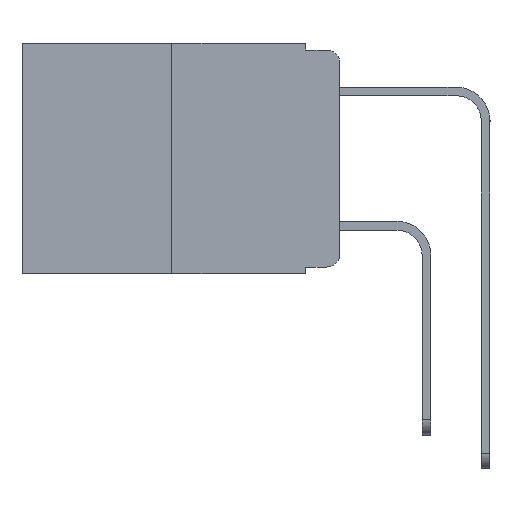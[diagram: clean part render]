
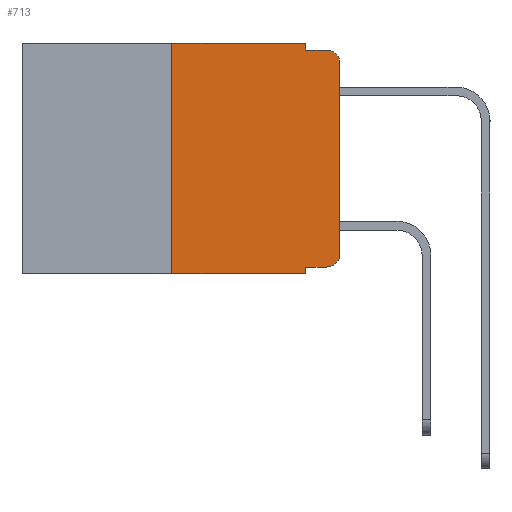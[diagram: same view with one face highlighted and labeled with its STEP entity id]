
A CAD part, left-side view. The second image highlights one B-rep face of the part: STEP entity #713.
In plain terms, the highlighted planar face has unit normal (-1, 0, 0).
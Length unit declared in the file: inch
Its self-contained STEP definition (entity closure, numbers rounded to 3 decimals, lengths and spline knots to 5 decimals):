
#25 = ORIENTED_EDGE ( 'NONE', *, *, #17406, .T. ) ;
#393 = EDGE_CURVE ( 'NONE', #20940, #3846, #13783, .T. ) ;
#543 = CARTESIAN_POINT ( 'NONE',  ( 0., 0.473, 0. ) ) ;
#713 = ADVANCED_FACE ( 'NONE', ( #4195 ), #10557, .F. ) ;
#765 = DIRECTION ( 'NONE',  ( -1., 0., 0. ) ) ;
#859 = ORIENTED_EDGE ( 'NONE', *, *, #20865, .F. ) ;
#892 = ORIENTED_EDGE ( 'NONE', *, *, #6324, .T. ) ;
#1026 = LINE ( 'NONE', #543, #13384 ) ;
#1221 = ORIENTED_EDGE ( 'NONE', *, *, #4015, .F. ) ;
#1346 = ORIENTED_EDGE ( 'NONE', *, *, #21997, .F. ) ;
#1424 = DIRECTION ( 'NONE',  ( 0., 0., -1. ) ) ;
#1643 = DIRECTION ( 'NONE',  ( 0., 0., -1. ) ) ;
#2556 = VERTEX_POINT ( 'NONE', #21588 ) ;
#2758 = VERTEX_POINT ( 'NONE', #13600 ) ;
#3079 = VERTEX_POINT ( 'NONE', #9327 ) ;
#3187 = VECTOR ( 'NONE', #20408, 39.37008 ) ;
#3202 = LINE ( 'NONE', #10182, #21230 ) ;
#3532 = VECTOR ( 'NONE', #13570, 39.37008 ) ;
#3764 = AXIS2_PLACEMENT_3D ( 'NONE', #10603, #13930, #14072 ) ;
#3846 = VERTEX_POINT ( 'NONE', #9689 ) ;
#4015 = EDGE_CURVE ( 'NONE', #3846, #3079, #12019, .T. ) ;
#4066 = LINE ( 'NONE', #11820, #3532 ) ;
#4195 = FACE_OUTER_BOUND ( 'NONE', #10237, .T. ) ;
#5270 = ORIENTED_EDGE ( 'NONE', *, *, #11207, .F. ) ;
#6020 = ORIENTED_EDGE ( 'NONE', *, *, #11349, .T. ) ;
#6324 = EDGE_CURVE ( 'NONE', #22658, #3079, #13782, .T. ) ;
#7052 = ORIENTED_EDGE ( 'NONE', *, *, #19728, .T. ) ;
#7058 = AXIS2_PLACEMENT_3D ( 'NONE', #22549, #12137, #1643 ) ;
#7547 = EDGE_CURVE ( 'NONE', #2758, #22658, #11817, .T. ) ;
#7906 = DIRECTION ( 'NONE',  ( 0., 0., 1. ) ) ;
#8142 = CARTESIAN_POINT ( 'NONE',  ( 0., 0.473, -0.343 ) ) ;
#8443 = DIRECTION ( 'NONE',  ( 0., -1., 0. ) ) ;
#8956 = ORIENTED_EDGE ( 'NONE', *, *, #393, .F. ) ;
#9171 = VECTOR ( 'NONE', #16840, 39.37008 ) ;
#9327 = CARTESIAN_POINT ( 'NONE',  ( 0., 0.02, -0.01 ) ) ;
#9527 = ORIENTED_EDGE ( 'NONE', *, *, #7547, .T. ) ;
#9666 = CARTESIAN_POINT ( 'NONE',  ( 0., 0., 0. ) ) ;
#9689 = CARTESIAN_POINT ( 'NONE',  ( 0., 0.051, -0.01 ) ) ;
#9865 = CARTESIAN_POINT ( 'NONE',  ( 0., 0.051, -0.333 ) ) ;
#10182 = CARTESIAN_POINT ( 'NONE',  ( 0., 0.051, 0. ) ) ;
#10237 = EDGE_LOOP ( 'NONE', ( #9527, #892, #1221, #8956, #5270, #1346, #6020, #859, #7052, #25 ) ) ;
#10557 = PLANE ( 'NONE',  #3764 ) ;
#10603 = CARTESIAN_POINT ( 'NONE',  ( 0., 0.473, 0. ) ) ;
#11193 = LINE ( 'NONE', #8142, #20529 ) ;
#11207 = EDGE_CURVE ( 'NONE', #12056, #20940, #1026, .T. ) ;
#11316 = CARTESIAN_POINT ( 'NONE',  ( 0., 0.02, -0.03 ) ) ;
#11349 = EDGE_CURVE ( 'NONE', #18081, #21793, #11193, .T. ) ;
#11817 = LINE ( 'NONE', #9666, #20598 ) ;
#11820 = CARTESIAN_POINT ( 'NONE',  ( 0., 0.051, -0.333 ) ) ;
#12019 = LINE ( 'NONE', #18952, #12558 ) ;
#12056 = VERTEX_POINT ( 'NONE', #18732 ) ;
#12137 = DIRECTION ( 'NONE',  ( -1., 0., 0. ) ) ;
#12558 = VECTOR ( 'NONE', #8443, 39.37008 ) ;
#13052 = DIRECTION ( 'NONE',  ( 0., 0., -1. ) ) ;
#13384 = VECTOR ( 'NONE', #14701, 39.37008 ) ;
#13443 = VERTEX_POINT ( 'NONE', #9865 ) ;
#13536 = CARTESIAN_POINT ( 'NONE',  ( 0., 0.051, 0. ) ) ;
#13570 = DIRECTION ( 'NONE',  ( 0., -1., 0. ) ) ;
#13600 = CARTESIAN_POINT ( 'NONE',  ( 0., 0., -0.313 ) ) ;
#13782 = CIRCLE ( 'NONE', #20558, 0.02 ) ;
#13783 = LINE ( 'NONE', #13536, #9171 ) ;
#13930 = DIRECTION ( 'NONE',  ( 1., 0., 0. ) ) ;
#14072 = DIRECTION ( 'NONE',  ( 0., 0., -1. ) ) ;
#14251 = CARTESIAN_POINT ( 'NONE',  ( 0., 0.25, -0.343 ) ) ;
#14572 = CARTESIAN_POINT ( 'NONE',  ( 0., 0.051, -0.343 ) ) ;
#14701 = DIRECTION ( 'NONE',  ( 0., -1., 0. ) ) ;
#15676 = CARTESIAN_POINT ( 'NONE',  ( 0., 0.051, 0. ) ) ;
#16149 = CIRCLE ( 'NONE', #7058, 0.02 ) ;
#16840 = DIRECTION ( 'NONE',  ( 0., 0., -1. ) ) ;
#17406 = EDGE_CURVE ( 'NONE', #2556, #2758, #16149, .T. ) ;
#17735 = LINE ( 'NONE', #18660, #3187 ) ;
#18081 = VERTEX_POINT ( 'NONE', #14251 ) ;
#18660 = CARTESIAN_POINT ( 'NONE',  ( 0., 0.25, 0. ) ) ;
#18732 = CARTESIAN_POINT ( 'NONE',  ( 0., 0.25, 0. ) ) ;
#18952 = CARTESIAN_POINT ( 'NONE',  ( 0., 0.051, -0.01 ) ) ;
#19728 = EDGE_CURVE ( 'NONE', #13443, #2556, #4066, .T. ) ;
#20393 = DIRECTION ( 'NONE',  ( 0., -1., 0. ) ) ;
#20408 = DIRECTION ( 'NONE',  ( 0., 0., 1. ) ) ;
#20529 = VECTOR ( 'NONE', #20393, 39.37008 ) ;
#20558 = AXIS2_PLACEMENT_3D ( 'NONE', #11316, #765, #13052 ) ;
#20598 = VECTOR ( 'NONE', #7906, 39.37008 ) ;
#20668 = CARTESIAN_POINT ( 'NONE',  ( 0., 0., -0.03 ) ) ;
#20865 = EDGE_CURVE ( 'NONE', #13443, #21793, #3202, .T. ) ;
#20940 = VERTEX_POINT ( 'NONE', #15676 ) ;
#21230 = VECTOR ( 'NONE', #1424, 39.37008 ) ;
#21588 = CARTESIAN_POINT ( 'NONE',  ( 0., 0.02, -0.333 ) ) ;
#21793 = VERTEX_POINT ( 'NONE', #14572 ) ;
#21997 = EDGE_CURVE ( 'NONE', #18081, #12056, #17735, .T. ) ;
#22549 = CARTESIAN_POINT ( 'NONE',  ( 0., 0.02, -0.313 ) ) ;
#22658 = VERTEX_POINT ( 'NONE', #20668 ) ;
